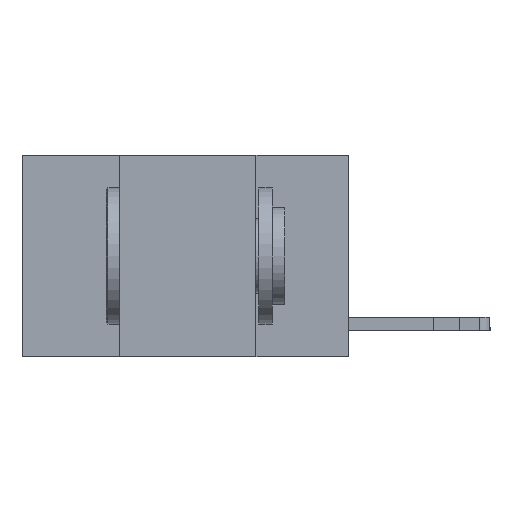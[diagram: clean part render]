
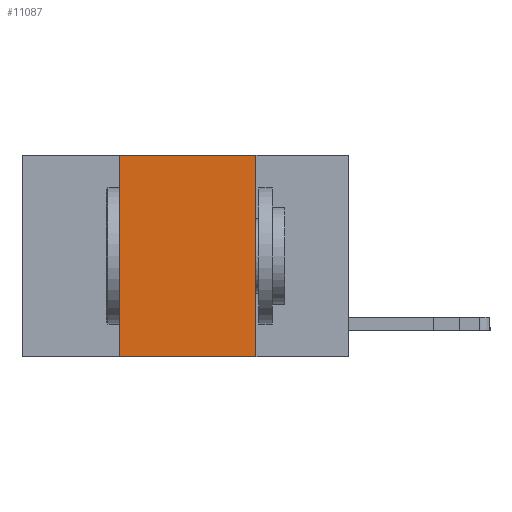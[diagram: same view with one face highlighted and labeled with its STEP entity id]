
A CAD part, left-side view. The second image highlights one B-rep face of the part: STEP entity #11087.
In plain terms, the highlighted planar face has unit normal (-1, 0, 0).
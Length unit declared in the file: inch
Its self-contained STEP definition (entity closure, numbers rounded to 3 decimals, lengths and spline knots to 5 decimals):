
#477 = EDGE_CURVE ( 'NONE', #19249, #24558, #16899, .T. ) ;
#656 = DIRECTION ( 'NONE',  ( 0., -1., 0. ) ) ;
#920 = AXIS2_PLACEMENT_3D ( 'NONE', #20463, #24093, #2572 ) ;
#1254 = CARTESIAN_POINT ( 'NONE',  ( 0., 0.42, 0. ) ) ;
#1479 = LINE ( 'NONE', #9586, #12015 ) ;
#1643 = DIRECTION ( 'NONE',  ( 0., 0., 1. ) ) ;
#2572 = DIRECTION ( 'NONE',  ( 0., 0., -1. ) ) ;
#3076 = CARTESIAN_POINT ( 'NONE',  ( 0., 0.42, 0. ) ) ;
#5624 = DIRECTION ( 'NONE',  ( 0., -1., 0. ) ) ;
#5837 = VECTOR ( 'NONE', #5624, 39.37008 ) ;
#6500 = PLANE ( 'NONE',  #920 ) ;
#6737 = VECTOR ( 'NONE', #1643, 39.37008 ) ;
#6740 = EDGE_CURVE ( 'NONE', #7396, #8290, #21453, .T. ) ;
#6833 = ORIENTED_EDGE ( 'NONE', *, *, #24368, .F. ) ;
#7396 = VERTEX_POINT ( 'NONE', #3076 ) ;
#7919 = CARTESIAN_POINT ( 'NONE',  ( 0., 0.17, -0.37 ) ) ;
#8290 = VERTEX_POINT ( 'NONE', #20184 ) ;
#9586 = CARTESIAN_POINT ( 'NONE',  ( 0., 0.17, 0. ) ) ;
#11087 = ADVANCED_FACE ( 'NONE', ( #20737 ), #6500, .F. ) ;
#11638 = CARTESIAN_POINT ( 'NONE',  ( 0., 0.6, 0. ) ) ;
#11803 = ORIENTED_EDGE ( 'NONE', *, *, #6740, .F. ) ;
#12015 = VECTOR ( 'NONE', #21500, 39.37008 ) ;
#12814 = EDGE_CURVE ( 'NONE', #8290, #24558, #1479, .T. ) ;
#13177 = LINE ( 'NONE', #1254, #6737 ) ;
#16308 = VECTOR ( 'NONE', #656, 39.37008 ) ;
#16899 = LINE ( 'NONE', #22870, #16308 ) ;
#19249 = VERTEX_POINT ( 'NONE', #19496 ) ;
#19496 = CARTESIAN_POINT ( 'NONE',  ( 0., 0.42, -0.37 ) ) ;
#20059 = ORIENTED_EDGE ( 'NONE', *, *, #12814, .F. ) ;
#20184 = CARTESIAN_POINT ( 'NONE',  ( 0., 0.17, 0. ) ) ;
#20463 = CARTESIAN_POINT ( 'NONE',  ( 0., 0.6, 0. ) ) ;
#20737 = FACE_OUTER_BOUND ( 'NONE', #23513, .T. ) ;
#21453 = LINE ( 'NONE', #11638, #5837 ) ;
#21500 = DIRECTION ( 'NONE',  ( 0., 0., -1. ) ) ;
#22870 = CARTESIAN_POINT ( 'NONE',  ( 0., 0.6, -0.37 ) ) ;
#23468 = ORIENTED_EDGE ( 'NONE', *, *, #477, .T. ) ;
#23513 = EDGE_LOOP ( 'NONE', ( #20059, #11803, #6833, #23468 ) ) ;
#24093 = DIRECTION ( 'NONE',  ( 1., 0., 0. ) ) ;
#24368 = EDGE_CURVE ( 'NONE', #19249, #7396, #13177, .T. ) ;
#24558 = VERTEX_POINT ( 'NONE', #7919 ) ;
